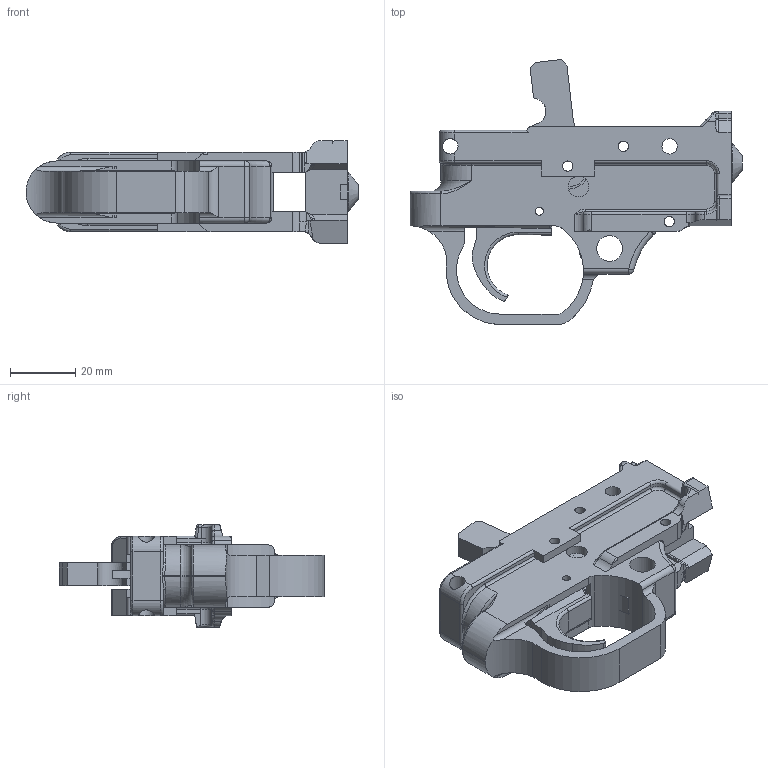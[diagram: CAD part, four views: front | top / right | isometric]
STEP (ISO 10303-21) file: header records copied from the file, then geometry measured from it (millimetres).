
FILE_DESCRIPTION((''),'2;1');
FILE_NAME('Trigger Group Complete.stp','2012-02-05T17:23:26',('Bob Clark'),(''),'Autodesk Inventor 2011','Autodesk Inventor 2011','');
FILE_SCHEMA(('AUTOMOTIVE_DESIGN { 1 0 10303 214 1 1 1 1 }'));
Length unit declared in the file: inch
Products named in the file (6): Trigger Group Complete; Trigger Housing; Trigger; Hammer; Hammer Bushing; Sear
Assembly tree (6 placements, depth 2):
  Trigger Group Complete
    Trigger Housing
    Trigger
    Hammer
    Hammer Bushing  x2
    Sear
Bounding box: 102.03 x 81.46 x 31.6 mm (x, y, z)
Volume: 46005.5 mm3; surface area: 26318.8 mm2
Topology: 6 solids, 6 shells, 364 faces, 1003 edges, 637 vertices
Faces by surface type: plane 157, cylinder 150, torus 31, bspline 19, sphere 6, cone 1
Full cylindrical faces by diameter (mm): 2.159 x2, 2.438 x2, 3.175 x8, 3.2 x1, 3.344 x1, 3.759 x1, 3.975 x2, 4.763 x3, 4.877 x1, 5.461 x1, 5.486 x2, 6.35 x1, 7.823 x2, 7.938 x1, 12.192 x1, 12.7 x2
Entity records: 12218 total; most frequent: CARTESIAN_POINT 2937, DIRECTION 1910, ORIENTED_EDGE 1888, EDGE_CURVE 944, AXIS2_PLACEMENT_3D 694, VERTEX_POINT 618, VECTOR 522, LINE 522
